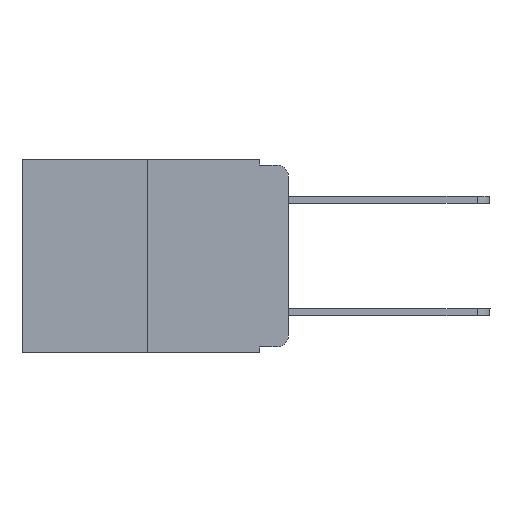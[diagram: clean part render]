
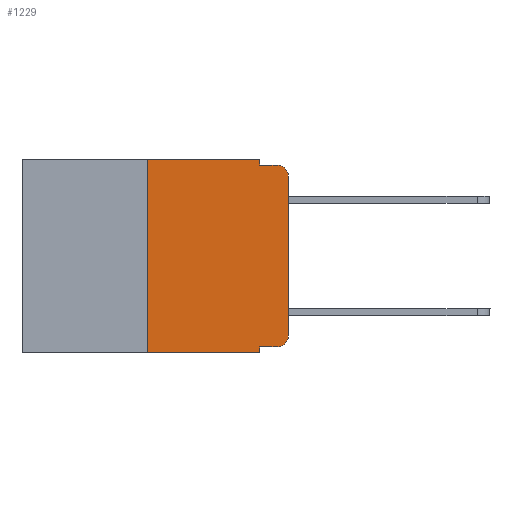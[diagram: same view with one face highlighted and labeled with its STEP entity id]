
A CAD part, left-side view. The second image highlights one B-rep face of the part: STEP entity #1229.
In plain terms, the highlighted planar face has unit normal (-1, 0, 0).
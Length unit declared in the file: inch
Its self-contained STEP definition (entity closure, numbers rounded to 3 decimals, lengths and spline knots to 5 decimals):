
#252 = VERTEX_POINT ( 'NONE', #22320 ) ;
#257 = CARTESIAN_POINT ( 'NONE',  ( 0., 0., -0.313 ) ) ;
#279 = CARTESIAN_POINT ( 'NONE',  ( 0., 0.02, -0.01 ) ) ;
#668 = VECTOR ( 'NONE', #8203, 39.37008 ) ;
#823 = EDGE_CURVE ( 'NONE', #252, #1764, #16142, .T. ) ;
#1229 = ADVANCED_FACE ( 'NONE', ( #13398 ), #1957, .F. ) ;
#1290 = CARTESIAN_POINT ( 'NONE',  ( 0., 0.051, 0. ) ) ;
#1438 = LINE ( 'NONE', #6875, #16605 ) ;
#1463 = VERTEX_POINT ( 'NONE', #257 ) ;
#1629 = DIRECTION ( 'NONE',  ( 1., 0., 0. ) ) ;
#1713 = CARTESIAN_POINT ( 'NONE',  ( 0., 0.25, -0.343 ) ) ;
#1764 = VERTEX_POINT ( 'NONE', #14323 ) ;
#1772 = DIRECTION ( 'NONE',  ( 0., 0., 1. ) ) ;
#1957 = PLANE ( 'NONE',  #12460 ) ;
#2119 = ORIENTED_EDGE ( 'NONE', *, *, #15850, .F. ) ;
#2710 = DIRECTION ( 'NONE',  ( 0., 0., 1. ) ) ;
#3403 = CIRCLE ( 'NONE', #7628, 0.02 ) ;
#3548 = EDGE_CURVE ( 'NONE', #21357, #17357, #24159, .T. ) ;
#3732 = DIRECTION ( 'NONE',  ( 0., 0., -1. ) ) ;
#3849 = CARTESIAN_POINT ( 'NONE',  ( 0., 0.051, -0.01 ) ) ;
#4258 = ORIENTED_EDGE ( 'NONE', *, *, #13172, .T. ) ;
#5545 = VECTOR ( 'NONE', #6855, 39.37008 ) ;
#6054 = LINE ( 'NONE', #1290, #10328 ) ;
#6152 = DIRECTION ( 'NONE',  ( 0., -1., 0. ) ) ;
#6309 = ORIENTED_EDGE ( 'NONE', *, *, #9895, .T. ) ;
#6312 = CIRCLE ( 'NONE', #12271, 0.02 ) ;
#6486 = ORIENTED_EDGE ( 'NONE', *, *, #15246, .F. ) ;
#6550 = DIRECTION ( 'NONE',  ( -1., 0., 0. ) ) ;
#6855 = DIRECTION ( 'NONE',  ( 0., -1., 0. ) ) ;
#6875 = CARTESIAN_POINT ( 'NONE',  ( 0., 0.051, 0. ) ) ;
#7178 = CARTESIAN_POINT ( 'NONE',  ( 0., 0.051, -0.01 ) ) ;
#7628 = AXIS2_PLACEMENT_3D ( 'NONE', #19354, #9647, #19234 ) ;
#8203 = DIRECTION ( 'NONE',  ( 0., -1., 0. ) ) ;
#8429 = CARTESIAN_POINT ( 'NONE',  ( 0., 0.02, -0.03 ) ) ;
#8473 = CARTESIAN_POINT ( 'NONE',  ( 0., 0.051, -0.333 ) ) ;
#9066 = CARTESIAN_POINT ( 'NONE',  ( 0., 0.051, -0.333 ) ) ;
#9261 = DIRECTION ( 'NONE',  ( 0., 0., -1. ) ) ;
#9647 = DIRECTION ( 'NONE',  ( -1., 0., 0. ) ) ;
#9895 = EDGE_CURVE ( 'NONE', #14717, #21575, #6312, .T. ) ;
#10137 = EDGE_CURVE ( 'NONE', #1463, #14717, #11758, .T. ) ;
#10328 = VECTOR ( 'NONE', #9261, 39.37008 ) ;
#10504 = VECTOR ( 'NONE', #16838, 39.37008 ) ;
#10603 = VECTOR ( 'NONE', #2710, 39.37008 ) ;
#10734 = VERTEX_POINT ( 'NONE', #17107 ) ;
#11348 = ORIENTED_EDGE ( 'NONE', *, *, #14271, .F. ) ;
#11758 = LINE ( 'NONE', #17306, #19613 ) ;
#11835 = CARTESIAN_POINT ( 'NONE',  ( 0., 0.473, -0.343 ) ) ;
#12271 = AXIS2_PLACEMENT_3D ( 'NONE', #8429, #6550, #14340 ) ;
#12460 = AXIS2_PLACEMENT_3D ( 'NONE', #15362, #1629, #3732 ) ;
#12542 = LINE ( 'NONE', #9066, #5545 ) ;
#12578 = ORIENTED_EDGE ( 'NONE', *, *, #10137, .T. ) ;
#12728 = DIRECTION ( 'NONE',  ( 0., 0., -1. ) ) ;
#13030 = EDGE_CURVE ( 'NONE', #19546, #10734, #12542, .T. ) ;
#13172 = EDGE_CURVE ( 'NONE', #10734, #1463, #3403, .T. ) ;
#13398 = FACE_OUTER_BOUND ( 'NONE', #19223, .T. ) ;
#14080 = ORIENTED_EDGE ( 'NONE', *, *, #3548, .T. ) ;
#14271 = EDGE_CURVE ( 'NONE', #21357, #252, #19065, .T. ) ;
#14323 = CARTESIAN_POINT ( 'NONE',  ( 0., 0.051, 0. ) ) ;
#14340 = DIRECTION ( 'NONE',  ( 0., 0., -1. ) ) ;
#14650 = CARTESIAN_POINT ( 'NONE',  ( 0., 0.25, 0. ) ) ;
#14717 = VERTEX_POINT ( 'NONE', #16098 ) ;
#15246 = EDGE_CURVE ( 'NONE', #19546, #17357, #1438, .T. ) ;
#15344 = LINE ( 'NONE', #7178, #10504 ) ;
#15362 = CARTESIAN_POINT ( 'NONE',  ( 0., 0.473, 0. ) ) ;
#15850 = EDGE_CURVE ( 'NONE', #23897, #21575, #15344, .T. ) ;
#16098 = CARTESIAN_POINT ( 'NONE',  ( 0., 0., -0.03 ) ) ;
#16142 = LINE ( 'NONE', #23648, #668 ) ;
#16605 = VECTOR ( 'NONE', #12728, 39.37008 ) ;
#16838 = DIRECTION ( 'NONE',  ( 0., -1., 0. ) ) ;
#17107 = CARTESIAN_POINT ( 'NONE',  ( 0., 0.02, -0.333 ) ) ;
#17306 = CARTESIAN_POINT ( 'NONE',  ( 0., 0., 0. ) ) ;
#17357 = VERTEX_POINT ( 'NONE', #23071 ) ;
#18442 = VECTOR ( 'NONE', #6152, 39.37008 ) ;
#19065 = LINE ( 'NONE', #14650, #10603 ) ;
#19149 = ORIENTED_EDGE ( 'NONE', *, *, #823, .F. ) ;
#19223 = EDGE_LOOP ( 'NONE', ( #12578, #6309, #2119, #24679, #19149, #11348, #14080, #6486, #22098, #4258 ) ) ;
#19234 = DIRECTION ( 'NONE',  ( 0., 0., -1. ) ) ;
#19354 = CARTESIAN_POINT ( 'NONE',  ( 0., 0.02, -0.313 ) ) ;
#19546 = VERTEX_POINT ( 'NONE', #8473 ) ;
#19613 = VECTOR ( 'NONE', #1772, 39.37008 ) ;
#20253 = EDGE_CURVE ( 'NONE', #1764, #23897, #6054, .T. ) ;
#21357 = VERTEX_POINT ( 'NONE', #1713 ) ;
#21575 = VERTEX_POINT ( 'NONE', #279 ) ;
#22098 = ORIENTED_EDGE ( 'NONE', *, *, #13030, .T. ) ;
#22320 = CARTESIAN_POINT ( 'NONE',  ( 0., 0.25, 0. ) ) ;
#23071 = CARTESIAN_POINT ( 'NONE',  ( 0., 0.051, -0.343 ) ) ;
#23648 = CARTESIAN_POINT ( 'NONE',  ( 0., 0.473, 0. ) ) ;
#23897 = VERTEX_POINT ( 'NONE', #3849 ) ;
#24159 = LINE ( 'NONE', #11835, #18442 ) ;
#24679 = ORIENTED_EDGE ( 'NONE', *, *, #20253, .F. ) ;
